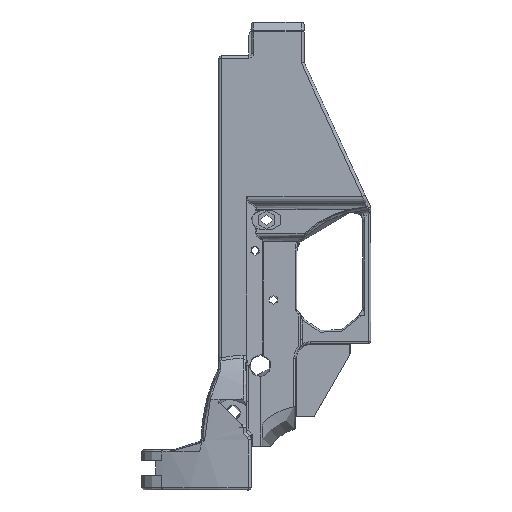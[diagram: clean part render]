
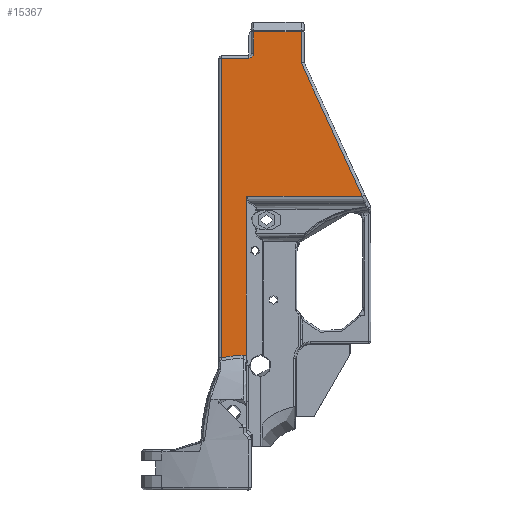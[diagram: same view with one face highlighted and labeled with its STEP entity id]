
A CAD part, left-side view. The second image highlights one B-rep face of the part: STEP entity #15367.
In plain terms, the highlighted planar face has unit normal (-1, 0, 0).
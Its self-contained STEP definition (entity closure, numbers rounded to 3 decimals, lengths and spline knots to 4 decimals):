
#222=ELLIPSE('',#16783,1.9201,1.636);
#401=PLANE('',#16781);
#1356=FACE_OUTER_BOUND('',#2316,.T.);
#2316=EDGE_LOOP('',(#12315,#12316,#12317,#12318,#12319,#12320,#12321,#12322,
#12323,#12324,#12325,#12326));
#3212=B_SPLINE_CURVE_WITH_KNOTS('',3,(#42844,#42845,#42846,#42847),
 .UNSPECIFIED.,.F.,.F.,(4,4),(-0.1434,0.),
 .UNSPECIFIED.);
#3213=B_SPLINE_CURVE_WITH_KNOTS('',3,(#42851,#42852,#42853,#42854,#42855,
#42856,#42857,#42858,#42859,#42860,#42861,#42862),.UNSPECIFIED.,.F.,.F.,
(4,2,2,2,2,4),(-0.117,-0.1147,-0.0798,
-0.057,-0.0072,0.),.UNSPECIFIED.);
#3869=CIRCLE('',#16782,0.08);
#4504=LINE('',#25503,#5272);
#4506=LINE('',#25534,#5274);
#4687=LINE('',#42796,#5455);
#4691=LINE('',#42834,#5459);
#4692=LINE('',#42838,#5460);
#4693=LINE('',#42840,#5461);
#4694=LINE('',#42849,#5462);
#4695=LINE('',#42863,#5463);
#5272=VECTOR('',#19008,0.3937);
#5274=VECTOR('',#19020,0.3937);
#5455=VECTOR('',#19869,0.3937);
#5459=VECTOR('',#19891,0.3937);
#5460=VECTOR('',#19894,0.3937);
#5461=VECTOR('',#19895,0.3937);
#5462=VECTOR('',#19898,1.6985);
#5463=VECTOR('',#19899,0.1181);
#6261=VERTEX_POINT('',#25500);
#6262=VERTEX_POINT('',#25502);
#6266=VERTEX_POINT('',#25532);
#6736=VERTEX_POINT('',#42794);
#6741=VERTEX_POINT('',#42833);
#6742=VERTEX_POINT('',#42835);
#6743=VERTEX_POINT('',#42837);
#6744=VERTEX_POINT('',#42839);
#6745=VERTEX_POINT('',#42841);
#6746=VERTEX_POINT('',#42843);
#6747=VERTEX_POINT('',#42848);
#6748=VERTEX_POINT('',#42850);
#8012=EDGE_CURVE('',#6261,#6262,#4504,.T.);
#8019=EDGE_CURVE('',#6266,#6261,#4506,.T.);
#8722=EDGE_CURVE('',#6736,#6266,#4687,.T.);
#8731=EDGE_CURVE('',#6741,#6736,#4691,.T.);
#8732=EDGE_CURVE('',#6742,#6741,#3869,.T.);
#8733=EDGE_CURVE('',#6743,#6742,#4692,.T.);
#8734=EDGE_CURVE('',#6744,#6743,#4693,.T.);
#8735=EDGE_CURVE('',#6745,#6744,#222,.T.);
#8736=EDGE_CURVE('',#6746,#6745,#3212,.T.);
#8737=EDGE_CURVE('',#6747,#6746,#4694,.T.);
#8738=EDGE_CURVE('',#6748,#6747,#3213,.T.);
#8739=EDGE_CURVE('',#6262,#6748,#4695,.T.);
#12315=ORIENTED_EDGE('',*,*,#8012,.F.);
#12316=ORIENTED_EDGE('',*,*,#8019,.F.);
#12317=ORIENTED_EDGE('',*,*,#8722,.F.);
#12318=ORIENTED_EDGE('',*,*,#8731,.F.);
#12319=ORIENTED_EDGE('',*,*,#8732,.F.);
#12320=ORIENTED_EDGE('',*,*,#8733,.F.);
#12321=ORIENTED_EDGE('',*,*,#8734,.F.);
#12322=ORIENTED_EDGE('',*,*,#8735,.F.);
#12323=ORIENTED_EDGE('',*,*,#8736,.F.);
#12324=ORIENTED_EDGE('',*,*,#8737,.F.);
#12325=ORIENTED_EDGE('',*,*,#8738,.F.);
#12326=ORIENTED_EDGE('',*,*,#8739,.F.);
#15367=ADVANCED_FACE('',(#1356),#401,.F.);
#16781=AXIS2_PLACEMENT_3D('',#42832,#19889,#19890);
#16782=AXIS2_PLACEMENT_3D('',#42836,#19892,#19893);
#16783=AXIS2_PLACEMENT_3D('',#42842,#19896,#19897);
#19008=DIRECTION('',(0.,-0.417,-0.909));
#19020=DIRECTION('',(0.,0.,-1.));
#19869=DIRECTION('',(0.,-1.,0.));
#19889=DIRECTION('center_axis',(1.,0.,0.));
#19890=DIRECTION('ref_axis',(0.,0.,
-1.));
#19891=DIRECTION('',(0.,0.,1.));
#19892=DIRECTION('center_axis',(-1.,0.,0.));
#19893=DIRECTION('ref_axis',(0.,-0.707,-0.707));
#19894=DIRECTION('',(0.,-1.,0.));
#19895=DIRECTION('',(0.,0.,1.));
#19896=DIRECTION('center_axis',(-1.,0.,0.));
#19897=DIRECTION('ref_axis',(0.,-0.984,-0.179));
#19898=DIRECTION('',(0.,0.,-1.));
#19899=DIRECTION('',(0.,1.,0.));
#25500=CARTESIAN_POINT('',(-0.731,-0.0727,2.8507));
#25502=CARTESIAN_POINT('',(-0.731,-1.118,0.5717));
#25503=CARTESIAN_POINT('',(-0.731,-1.4648,-0.1846));
#25532=CARTESIAN_POINT('',(-0.731,-0.0728,3.3816));
#25534=CARTESIAN_POINT('',(-0.731,-0.0727,-0.2092));
#42794=CARTESIAN_POINT('',(-0.731,0.7372,3.3816));
#42796=CARTESIAN_POINT('',(-0.731,0.7121,3.3816));
#42832=CARTESIAN_POINT('Origin',(-0.731,0.68,-3.6849));
#42833=CARTESIAN_POINT('',(-0.731,0.7373,3.0095));
#42834=CARTESIAN_POINT('',(-0.731,0.7373,-0.0118));
#42835=CARTESIAN_POINT('',(-0.731,0.8173,2.9295));
#42836=CARTESIAN_POINT('Origin',(-0.731,0.8173,3.0095));
#42837=CARTESIAN_POINT('',(-0.731,1.2902,2.9295));
#42838=CARTESIAN_POINT('',(-0.731,0.7441,2.9295));
#42839=CARTESIAN_POINT('',(-0.731,1.2902,-2.1813));
#42840=CARTESIAN_POINT('',(-0.731,1.2902,-3.1756));
#42841=CARTESIAN_POINT('',(-0.731,0.9158,-2.1342));
#42842=CARTESIAN_POINT('Origin',(-0.731,0.7244,-3.7785));
#42843=CARTESIAN_POINT('',(-0.731,0.8628,-2.151));
#42844=CARTESIAN_POINT('Ctrl Pts',(-0.731,0.8629,
-2.151));
#42845=CARTESIAN_POINT('Ctrl Pts',(-0.731,0.8784,
-2.1404));
#42846=CARTESIAN_POINT('Ctrl Pts',(-0.731,0.8969,
-2.1335));
#42847=CARTESIAN_POINT('Ctrl Pts',(-0.731,0.9158,
-2.1342));
#42848=CARTESIAN_POINT('',(-0.731,0.8628,0.5319));
#42849=CARTESIAN_POINT('',(-0.731,0.8628,-2.5001));
#42850=CARTESIAN_POINT('',(-0.731,0.8546,0.5717));
#42851=CARTESIAN_POINT('Ctrl Pts',(-0.731,0.8546,
0.5717));
#42852=CARTESIAN_POINT('Ctrl Pts',(-0.731,0.8546,
0.5716));
#42853=CARTESIAN_POINT('Ctrl Pts',(-0.731,0.8546,
0.5716));
#42854=CARTESIAN_POINT('Ctrl Pts',(-0.731,0.855,
0.5706));
#42855=CARTESIAN_POINT('Ctrl Pts',(-0.731,0.8564,
0.5674));
#42856=CARTESIAN_POINT('Ctrl Pts',(-0.731,0.8587,
0.5601));
#42857=CARTESIAN_POINT('Ctrl Pts',(-0.731,0.8595,
0.5572));
#42858=CARTESIAN_POINT('Ctrl Pts',(-0.731,0.8617,
0.5478));
#42859=CARTESIAN_POINT('Ctrl Pts',(-0.731,0.8626,
0.5413));
#42860=CARTESIAN_POINT('Ctrl Pts',(-0.731,0.8628,
0.5338));
#42861=CARTESIAN_POINT('Ctrl Pts',(-0.731,0.8628,
0.5329));
#42862=CARTESIAN_POINT('Ctrl Pts',(-0.731,0.8628,
0.5319));
#42863=CARTESIAN_POINT('',(-0.731,1.0895,0.5717));
